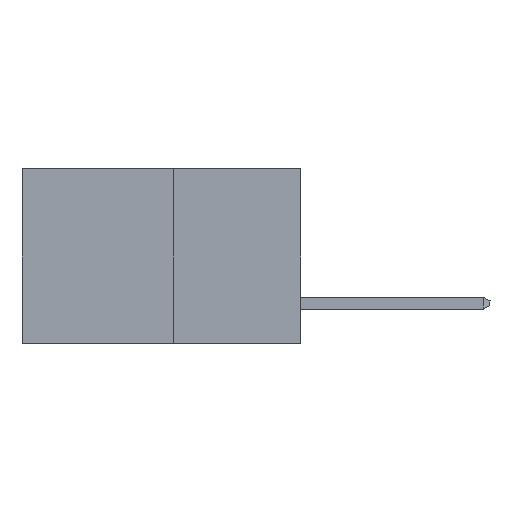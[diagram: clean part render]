
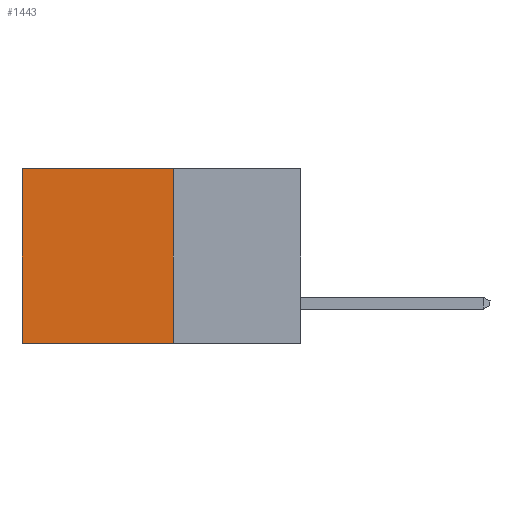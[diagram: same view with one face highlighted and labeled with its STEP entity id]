
A CAD part, left-side view. The second image highlights one B-rep face of the part: STEP entity #1443.
In plain terms, the highlighted planar face has unit normal (-1, 0, 0).
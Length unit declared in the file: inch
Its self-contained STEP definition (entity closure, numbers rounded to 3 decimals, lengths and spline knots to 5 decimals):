
#147 = DIRECTION ( 'NONE',  ( 0., 0., -1. ) ) ;
#1443 = ADVANCED_FACE ( 'NONE', ( #15362 ), #24444, .F. ) ;
#1690 = ORIENTED_EDGE ( 'NONE', *, *, #27667, .F. ) ;
#2669 = CARTESIAN_POINT ( 'NONE',  ( 0.277, 0.27, -0.37 ) ) ;
#3433 = LINE ( 'NONE', #12814, #21479 ) ;
#6066 = VERTEX_POINT ( 'NONE', #28170 ) ;
#6367 = ORIENTED_EDGE ( 'NONE', *, *, #11197, .T. ) ;
#8508 = EDGE_CURVE ( 'NONE', #25116, #17353, #29061, .T. ) ;
#8873 = EDGE_LOOP ( 'NONE', ( #27876, #1690, #31418, #6367 ) ) ;
#10010 = CARTESIAN_POINT ( 'NONE',  ( 0.277, 0.59, -0.37 ) ) ;
#10728 = VECTOR ( 'NONE', #17574, 39.37008 ) ;
#11197 = EDGE_CURVE ( 'NONE', #22880, #25116, #23695, .T. ) ;
#12109 = DIRECTION ( 'NONE',  ( 1., 0., 0. ) ) ;
#12145 = CARTESIAN_POINT ( 'NONE',  ( 0.277, 0.27, -0.37 ) ) ;
#12559 = CARTESIAN_POINT ( 'NONE',  ( 0.277, 0.27, 0. ) ) ;
#12814 = CARTESIAN_POINT ( 'NONE',  ( 0.277, 0.27, -0.37 ) ) ;
#14364 = AXIS2_PLACEMENT_3D ( 'NONE', #12145, #12109, #147 ) ;
#15362 = FACE_OUTER_BOUND ( 'NONE', #8873, .T. ) ;
#15532 = EDGE_CURVE ( 'NONE', #22880, #6066, #3433, .T. ) ;
#15942 = CARTESIAN_POINT ( 'NONE',  ( 0.277, 0.59, -0.37 ) ) ;
#16984 = VECTOR ( 'NONE', #19880, 39.37008 ) ;
#17353 = VERTEX_POINT ( 'NONE', #10010 ) ;
#17574 = DIRECTION ( 'NONE',  ( 0., 1., 0. ) ) ;
#18443 = DIRECTION ( 'NONE',  ( 0., 0., -1. ) ) ;
#19880 = DIRECTION ( 'NONE',  ( 0., 1., 0. ) ) ;
#20107 = CARTESIAN_POINT ( 'NONE',  ( 0.277, 0.27, 0. ) ) ;
#20820 = CARTESIAN_POINT ( 'NONE',  ( 0.277, 0.59, 0. ) ) ;
#21479 = VECTOR ( 'NONE', #29803, 39.37008 ) ;
#22880 = VERTEX_POINT ( 'NONE', #20107 ) ;
#23695 = LINE ( 'NONE', #12559, #10728 ) ;
#24261 = VECTOR ( 'NONE', #18443, 39.37008 ) ;
#24444 = PLANE ( 'NONE',  #14364 ) ;
#25116 = VERTEX_POINT ( 'NONE', #20820 ) ;
#27667 = EDGE_CURVE ( 'NONE', #6066, #17353, #28946, .T. ) ;
#27876 = ORIENTED_EDGE ( 'NONE', *, *, #8508, .T. ) ;
#28170 = CARTESIAN_POINT ( 'NONE',  ( 0.277, 0.27, -0.37 ) ) ;
#28946 = LINE ( 'NONE', #2669, #16984 ) ;
#29061 = LINE ( 'NONE', #15942, #24261 ) ;
#29803 = DIRECTION ( 'NONE',  ( 0., 0., -1. ) ) ;
#31418 = ORIENTED_EDGE ( 'NONE', *, *, #15532, .F. ) ;
